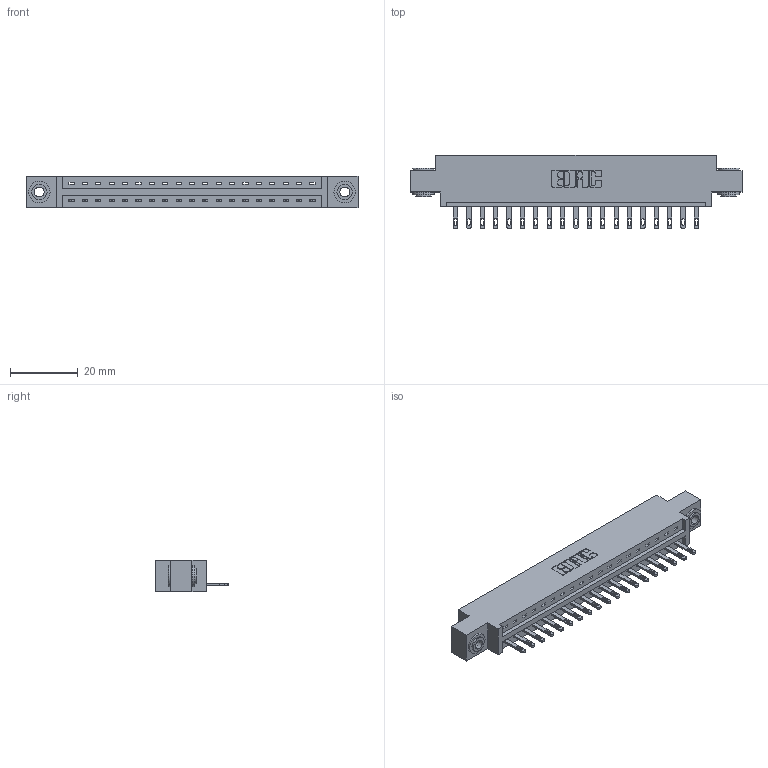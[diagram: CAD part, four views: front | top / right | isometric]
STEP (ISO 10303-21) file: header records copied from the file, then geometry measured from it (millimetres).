
FILE_DESCRIPTION (( 'STEP AP203' ), '1' );
FILE_NAME ('887-019-500-603.STEP', '2020-09-20T17:57:38', ( '' ), ( '' ), 'SwSTEP 2.0', 'SolidWorks 2020', '' );
FILE_SCHEMA (( 'CONFIG_CONTROL_DESIGN' ));
Length unit declared in the file: inch
Products named in the file (4): 887-019-500-603; 345-292-001_345-293-100; 837 Part_0.170 Offset - 0.156 Dia-TH; 345-250-002_345-250-002-102
Assembly tree (22 placements, depth 2):
  887-019-500-603
    837 Part_0.170 Offset - 0.156 Dia-TH
    345-292-001_345-293-100  x19
    345-250-002_345-250-002-102  x2
Bounding box: 98.3 x 21.85 x 9.4 mm (x, y, z)
Volume: 9842.3 mm3; surface area: 10416.4 mm2
Topology: 22 solids, 22 shells, 1258 faces, 3819 edges, 2542 vertices
Faces by surface type: plane 844, cylinder 406, cone 8
Entity records: 17810 total; most frequent: CARTESIAN_POINT 3078, ORIENTED_EDGE 3026, DIRECTION 2673, EDGE_CURVE 1513, LINE 1357, VECTOR 1357, VERTEX_POINT 1006, AXIS2_PLACEMENT_3D 658
